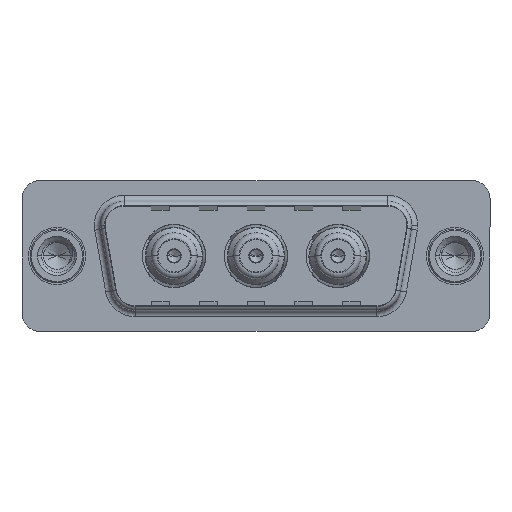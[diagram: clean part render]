
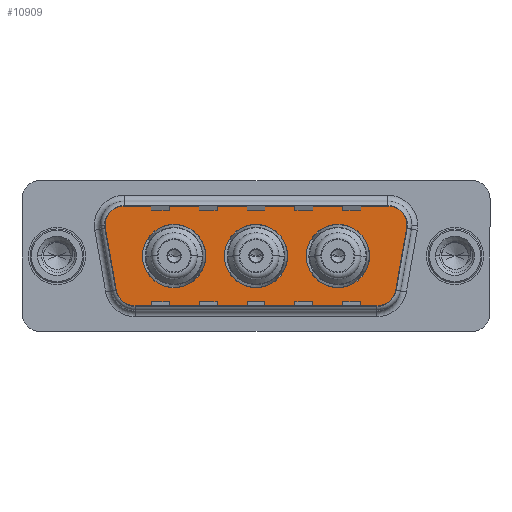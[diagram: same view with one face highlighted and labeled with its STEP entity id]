
A CAD part, top view. The second image highlights one B-rep face of the part: STEP entity #10909.
In plain terms, the highlighted planar face has unit normal (0, 0, 1).
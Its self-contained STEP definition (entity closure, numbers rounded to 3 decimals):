
#79 = EDGE_LOOP ( 'NONE', ( #11231, #1084 ) ) ;
#119 = LINE ( 'NONE', #16226, #7017 ) ;
#221 = CARTESIAN_POINT ( 'NONE',  ( 6.434, -4.9, 0. ) ) ;
#545 = CARTESIAN_POINT ( 'NONE',  ( 27.889, 2.9, 0. ) ) ;
#584 = DIRECTION ( 'NONE',  ( 1., 0., 0. ) ) ;
#709 = AXIS2_PLACEMENT_3D ( 'NONE', #7132, #16321, #8423 ) ;
#769 = ORIENTED_EDGE ( 'NONE', *, *, #13317, .T. ) ;
#1084 = ORIENTED_EDGE ( 'NONE', *, *, #1398, .F. ) ;
#1304 = ORIENTED_EDGE ( 'NONE', *, *, #1577, .T. ) ;
#1322 = EDGE_CURVE ( 'NONE', #8443, #6307, #16091, .T. ) ;
#1354 = CIRCLE ( 'NONE', #5628, 2.65 ) ;
#1398 = EDGE_CURVE ( 'NONE', #6066, #14803, #1480, .T. ) ;
#1480 = CIRCLE ( 'NONE', #13443, 2.65 ) ;
#1577 = EDGE_CURVE ( 'NONE', #16560, #5349, #7060, .T. ) ;
#1819 = AXIS2_PLACEMENT_3D ( 'NONE', #5663, #14811, #6986 ) ;
#1961 = DIRECTION ( 'NONE',  ( -1., 0., 0. ) ) ;
#2107 = CARTESIAN_POINT ( 'NONE',  ( 27.889, 4.9, 0. ) ) ;
#2133 = AXIS2_PLACEMENT_3D ( 'NONE', #3667, #12883, #5056 ) ;
#2307 = LINE ( 'NONE', #221, #16027 ) ;
#2357 = CARTESIAN_POINT ( 'NONE',  ( 23.5, 0., 0. ) ) ;
#2388 = EDGE_CURVE ( 'NONE', #2635, #2974, #17306, .T. ) ;
#2404 = VERTEX_POINT ( 'NONE', #14254 ) ;
#2406 = CARTESIAN_POINT ( 'NONE',  ( 28.836, -3.247, 0. ) ) ;
#2486 = DIRECTION ( 'NONE',  ( 0., 0., 1. ) ) ;
#2498 = AXIS2_PLACEMENT_3D ( 'NONE', #12039, #4202, #13399 ) ;
#2635 = VERTEX_POINT ( 'NONE', #8970 ) ;
#2673 = CIRCLE ( 'NONE', #8473, 2. ) ;
#2891 = CARTESIAN_POINT ( 'NONE',  ( 3.441, 2.553, 0. ) ) ;
#2974 = VERTEX_POINT ( 'NONE', #15444 ) ;
#3046 = PLANE ( 'NONE',  #709 ) ;
#3218 = CARTESIAN_POINT ( 'NONE',  ( 20.85, 0., 0. ) ) ;
#3402 = CARTESIAN_POINT ( 'NONE',  ( 26.15, 0., 0. ) ) ;
#3565 = DIRECTION ( 'NONE',  ( 0., 0., 1. ) ) ;
#3667 = CARTESIAN_POINT ( 'NONE',  ( 5.411, 2.9, 0. ) ) ;
#3790 = DIRECTION ( 'NONE',  ( 1., 0., 0. ) ) ;
#4202 = DIRECTION ( 'NONE',  ( 0., 0., 1. ) ) ;
#4245 = CARTESIAN_POINT ( 'NONE',  ( 6.434, -2.9, 0. ) ) ;
#4339 = FACE_OUTER_BOUND ( 'NONE', #16755, .T. ) ;
#4472 = EDGE_LOOP ( 'NONE', ( #11911, #4852 ) ) ;
#4566 = DIRECTION ( 'NONE',  ( 1., 0., 0. ) ) ;
#4852 = ORIENTED_EDGE ( 'NONE', *, *, #14531, .F. ) ;
#5056 = DIRECTION ( 'NONE',  ( 1., 0., 0. ) ) ;
#5102 = EDGE_CURVE ( 'NONE', #14532, #8443, #13326, .T. ) ;
#5117 = CARTESIAN_POINT ( 'NONE',  ( 16.65, 0., 0. ) ) ;
#5253 = EDGE_LOOP ( 'NONE', ( #10507, #14209 ) ) ;
#5349 = VERTEX_POINT ( 'NONE', #2406 ) ;
#5475 = CIRCLE ( 'NONE', #15692, 2.65 ) ;
#5628 = AXIS2_PLACEMENT_3D ( 'NONE', #2357, #11638, #3790 ) ;
#5663 = CARTESIAN_POINT ( 'NONE',  ( 9.8, 0., 0. ) ) ;
#5880 = CARTESIAN_POINT ( 'NONE',  ( 19.3, 0., 0. ) ) ;
#6022 = AXIS2_PLACEMENT_3D ( 'NONE', #7959, #6853, #11507 ) ;
#6066 = VERTEX_POINT ( 'NONE', #15892 ) ;
#6307 = VERTEX_POINT ( 'NONE', #11058 ) ;
#6324 = ORIENTED_EDGE ( 'NONE', *, *, #16211, .T. ) ;
#6853 = DIRECTION ( 'NONE',  ( 0., 0., 1. ) ) ;
#6986 = DIRECTION ( 'NONE',  ( 1., 0., 0. ) ) ;
#6989 = AXIS2_PLACEMENT_3D ( 'NONE', #10263, #7301, #15974 ) ;
#7017 = VECTOR ( 'NONE', #9638, 1000. ) ;
#7060 = CIRCLE ( 'NONE', #6989, 2. ) ;
#7132 = CARTESIAN_POINT ( 'NONE',  ( 26.866, -2.9, 0. ) ) ;
#7301 = DIRECTION ( 'NONE',  ( 0., 0., 1. ) ) ;
#7305 = EDGE_CURVE ( 'NONE', #15555, #7752, #1354, .T. ) ;
#7353 = AXIS2_PLACEMENT_3D ( 'NONE', #11409, #3565, #12777 ) ;
#7403 = DIRECTION ( 'NONE',  ( 0.174, 0.985, 0. ) ) ;
#7513 = EDGE_CURVE ( 'NONE', #14803, #6066, #9563, .T. ) ;
#7740 = EDGE_CURVE ( 'NONE', #10950, #10595, #2673, .T. ) ;
#7752 = VERTEX_POINT ( 'NONE', #3402 ) ;
#7764 = ORIENTED_EDGE ( 'NONE', *, *, #12083, .T. ) ;
#7851 = FACE_BOUND ( 'NONE', #4472, .T. ) ;
#7959 = CARTESIAN_POINT ( 'NONE',  ( 9.8, 0., 0. ) ) ;
#8112 = CARTESIAN_POINT ( 'NONE',  ( 29.859, 2.553, 0. ) ) ;
#8384 = EDGE_CURVE ( 'NONE', #7752, #15555, #5475, .T. ) ;
#8423 = DIRECTION ( 'NONE',  ( 1., 0., 0. ) ) ;
#8443 = VERTEX_POINT ( 'NONE', #16680 ) ;
#8473 = AXIS2_PLACEMENT_3D ( 'NONE', #545, #9991, #1961 ) ;
#8659 = FACE_BOUND ( 'NONE', #5253, .T. ) ;
#8714 = DIRECTION ( 'NONE',  ( 0., 0., 1. ) ) ;
#8970 = CARTESIAN_POINT ( 'NONE',  ( 12.45, 0., 0. ) ) ;
#9415 = VECTOR ( 'NONE', #7403, 1000. ) ;
#9563 = CIRCLE ( 'NONE', #2498, 2.65 ) ;
#9638 = DIRECTION ( 'NONE',  ( -1., 0., 0. ) ) ;
#9912 = AXIS2_PLACEMENT_3D ( 'NONE', #4245, #12575, #15424 ) ;
#9991 = DIRECTION ( 'NONE',  ( 0., 0., 1. ) ) ;
#10263 = CARTESIAN_POINT ( 'NONE',  ( 26.866, -2.9, 0. ) ) ;
#10358 = ORIENTED_EDGE ( 'NONE', *, *, #12445, .T. ) ;
#10507 = ORIENTED_EDGE ( 'NONE', *, *, #8384, .F. ) ;
#10595 = VERTEX_POINT ( 'NONE', #2107 ) ;
#10695 = CIRCLE ( 'NONE', #7353, 2. ) ;
#10909 = ADVANCED_FACE ( 'NONE', ( #11275, #8659, #7851, #4339 ), #3046, .T. ) ;
#10950 = VERTEX_POINT ( 'NONE', #16378 ) ;
#11058 = CARTESIAN_POINT ( 'NONE',  ( 6.434, -4.9, 0. ) ) ;
#11231 = ORIENTED_EDGE ( 'NONE', *, *, #7513, .F. ) ;
#11275 = FACE_BOUND ( 'NONE', #79, .T. ) ;
#11409 = CARTESIAN_POINT ( 'NONE',  ( 27.889, 2.9, 0. ) ) ;
#11507 = DIRECTION ( 'NONE',  ( 1., 0., 0. ) ) ;
#11638 = DIRECTION ( 'NONE',  ( 0., 0., 1. ) ) ;
#11911 = ORIENTED_EDGE ( 'NONE', *, *, #2388, .F. ) ;
#12038 = ORIENTED_EDGE ( 'NONE', *, *, #12912, .T. ) ;
#12039 = CARTESIAN_POINT ( 'NONE',  ( 16.65, 0., 0. ) ) ;
#12083 = EDGE_CURVE ( 'NONE', #2404, #14532, #13146, .T. ) ;
#12445 = EDGE_CURVE ( 'NONE', #5349, #12838, #16022, .T. ) ;
#12575 = DIRECTION ( 'NONE',  ( 0., 0., 1. ) ) ;
#12777 = DIRECTION ( 'NONE',  ( -1., 0., 0. ) ) ;
#12838 = VERTEX_POINT ( 'NONE', #8112 ) ;
#12883 = DIRECTION ( 'NONE',  ( 0., 0., 1. ) ) ;
#12912 = EDGE_CURVE ( 'NONE', #10595, #2404, #119, .T. ) ;
#13039 = CIRCLE ( 'NONE', #1819, 2.65 ) ;
#13146 = CIRCLE ( 'NONE', #2133, 2. ) ;
#13317 = EDGE_CURVE ( 'NONE', #6307, #16560, #2307, .T. ) ;
#13326 = LINE ( 'NONE', #15359, #16848 ) ;
#13399 = DIRECTION ( 'NONE',  ( 1., 0., 0. ) ) ;
#13443 = AXIS2_PLACEMENT_3D ( 'NONE', #5117, #2486, #4566 ) ;
#13649 = DIRECTION ( 'NONE',  ( 1., 0., 0. ) ) ;
#13696 = ORIENTED_EDGE ( 'NONE', *, *, #7740, .T. ) ;
#13903 = CARTESIAN_POINT ( 'NONE',  ( 29.859, 2.553, 0. ) ) ;
#14162 = ORIENTED_EDGE ( 'NONE', *, *, #5102, .T. ) ;
#14209 = ORIENTED_EDGE ( 'NONE', *, *, #7305, .F. ) ;
#14254 = CARTESIAN_POINT ( 'NONE',  ( 5.411, 4.9, 0. ) ) ;
#14531 = EDGE_CURVE ( 'NONE', #2974, #2635, #13039, .T. ) ;
#14532 = VERTEX_POINT ( 'NONE', #2891 ) ;
#14783 = CARTESIAN_POINT ( 'NONE',  ( 26.866, -4.9, 0. ) ) ;
#14803 = VERTEX_POINT ( 'NONE', #5880 ) ;
#14811 = DIRECTION ( 'NONE',  ( 0., 0., 1. ) ) ;
#15359 = CARTESIAN_POINT ( 'NONE',  ( 3.441, 2.553, 0. ) ) ;
#15424 = DIRECTION ( 'NONE',  ( -1., 0., 0. ) ) ;
#15444 = CARTESIAN_POINT ( 'NONE',  ( 7.15, 0., 0. ) ) ;
#15555 = VERTEX_POINT ( 'NONE', #3218 ) ;
#15692 = AXIS2_PLACEMENT_3D ( 'NONE', #16621, #8714, #584 ) ;
#15892 = CARTESIAN_POINT ( 'NONE',  ( 14., 0., 0. ) ) ;
#15909 = DIRECTION ( 'NONE',  ( 0.174, -0.985, 0. ) ) ;
#15974 = DIRECTION ( 'NONE',  ( 1., 0., 0. ) ) ;
#16022 = LINE ( 'NONE', #13903, #9415 ) ;
#16027 = VECTOR ( 'NONE', #13649, 1000. ) ;
#16091 = CIRCLE ( 'NONE', #9912, 2. ) ;
#16211 = EDGE_CURVE ( 'NONE', #12838, #10950, #10695, .T. ) ;
#16226 = CARTESIAN_POINT ( 'NONE',  ( 5.411, 4.9, 0. ) ) ;
#16321 = DIRECTION ( 'NONE',  ( 0., 0., 1. ) ) ;
#16378 = CARTESIAN_POINT ( 'NONE',  ( 29.889, 2.9, 0. ) ) ;
#16560 = VERTEX_POINT ( 'NONE', #14783 ) ;
#16621 = CARTESIAN_POINT ( 'NONE',  ( 23.5, 0., 0. ) ) ;
#16661 = ORIENTED_EDGE ( 'NONE', *, *, #1322, .T. ) ;
#16680 = CARTESIAN_POINT ( 'NONE',  ( 4.464, -3.247, 0. ) ) ;
#16755 = EDGE_LOOP ( 'NONE', ( #1304, #10358, #6324, #13696, #12038, #7764, #14162, #16661, #769 ) ) ;
#16848 = VECTOR ( 'NONE', #15909, 1000. ) ;
#17306 = CIRCLE ( 'NONE', #6022, 2.65 ) ;
